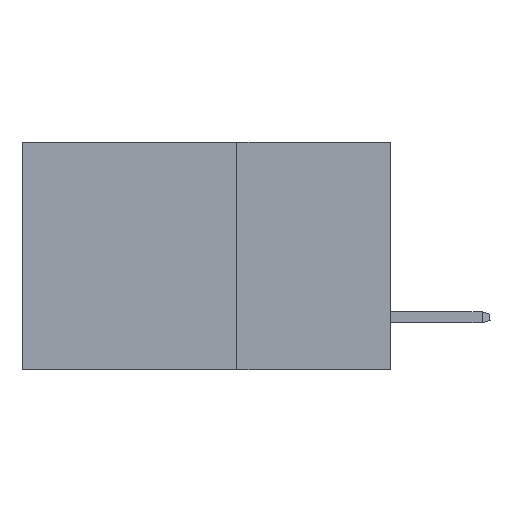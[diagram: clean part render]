
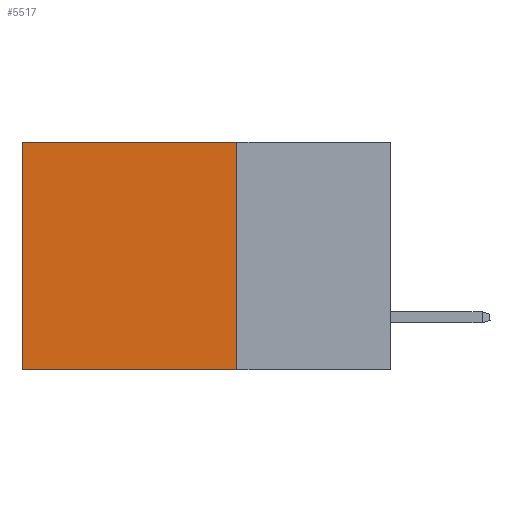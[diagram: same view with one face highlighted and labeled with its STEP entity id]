
A CAD part, left-side view. The second image highlights one B-rep face of the part: STEP entity #5517.
In plain terms, the highlighted planar face has unit normal (-1, 0, 0).
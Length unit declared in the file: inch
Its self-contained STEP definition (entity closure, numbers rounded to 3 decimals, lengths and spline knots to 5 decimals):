
#19 = CARTESIAN_POINT ( 'NONE',  ( 0.2875, 0.25, 0. ) ) ;
#413 = CARTESIAN_POINT ( 'NONE',  ( 0.2875, 0.6, 0. ) ) ;
#555 = EDGE_CURVE ( 'NONE', #2488, #6026, #2065, .T. ) ;
#1580 = CARTESIAN_POINT ( 'NONE',  ( 0.2875, 0.25, 0. ) ) ;
#1813 = EDGE_CURVE ( 'NONE', #6026, #4401, #10224, .T. ) ;
#2065 = LINE ( 'NONE', #19, #9450 ) ;
#2488 = VERTEX_POINT ( 'NONE', #1580 ) ;
#2762 = EDGE_CURVE ( 'NONE', #2488, #6608, #9129, .T. ) ;
#3122 = LINE ( 'NONE', #8510, #7788 ) ;
#3279 = CARTESIAN_POINT ( 'NONE',  ( 0.2875, 0.6, 0. ) ) ;
#3764 = DIRECTION ( 'NONE',  ( 0., 0., -1. ) ) ;
#3777 = DIRECTION ( 'NONE',  ( 1., 0., 0. ) ) ;
#3783 = PLANE ( 'NONE',  #11562 ) ;
#3830 = CARTESIAN_POINT ( 'NONE',  ( 0.2875, 0.25, 0. ) ) ;
#3907 = ORIENTED_EDGE ( 'NONE', *, *, #555, .T. ) ;
#3934 = CARTESIAN_POINT ( 'NONE',  ( 0.2875, 0.25, -0.37 ) ) ;
#4401 = VERTEX_POINT ( 'NONE', #11017 ) ;
#4527 = EDGE_LOOP ( 'NONE', ( #10083, #6797, #4543, #3907 ) ) ;
#4543 = ORIENTED_EDGE ( 'NONE', *, *, #2762, .F. ) ;
#5018 = DIRECTION ( 'NONE',  ( 0., 0., -1. ) ) ;
#5517 = ADVANCED_FACE ( 'NONE', ( #11875 ), #3783, .F. ) ;
#6026 = VERTEX_POINT ( 'NONE', #413 ) ;
#6608 = VERTEX_POINT ( 'NONE', #3934 ) ;
#6692 = VECTOR ( 'NONE', #9974, 39.37008 ) ;
#6797 = ORIENTED_EDGE ( 'NONE', *, *, #11015, .F. ) ;
#6953 = DIRECTION ( 'NONE',  ( 0., 1., 0. ) ) ;
#7788 = VECTOR ( 'NONE', #11133, 39.37008 ) ;
#7867 = VECTOR ( 'NONE', #5018, 39.37008 ) ;
#8510 = CARTESIAN_POINT ( 'NONE',  ( 0.2875, 0.25, -0.37 ) ) ;
#9129 = LINE ( 'NONE', #11119, #6692 ) ;
#9450 = VECTOR ( 'NONE', #6953, 39.37008 ) ;
#9974 = DIRECTION ( 'NONE',  ( 0., 0., -1. ) ) ;
#10083 = ORIENTED_EDGE ( 'NONE', *, *, #1813, .T. ) ;
#10224 = LINE ( 'NONE', #3279, #7867 ) ;
#11015 = EDGE_CURVE ( 'NONE', #6608, #4401, #3122, .T. ) ;
#11017 = CARTESIAN_POINT ( 'NONE',  ( 0.2875, 0.6, -0.37 ) ) ;
#11119 = CARTESIAN_POINT ( 'NONE',  ( 0.2875, 0.25, 0. ) ) ;
#11133 = DIRECTION ( 'NONE',  ( 0., 1., 0. ) ) ;
#11562 = AXIS2_PLACEMENT_3D ( 'NONE', #3830, #3777, #3764 ) ;
#11875 = FACE_OUTER_BOUND ( 'NONE', #4527, .T. ) ;
